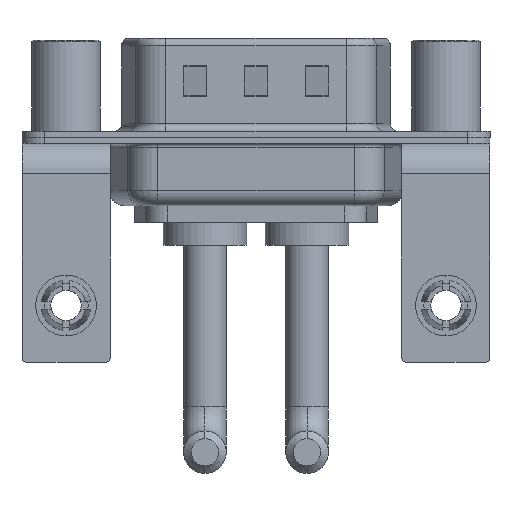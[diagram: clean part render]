
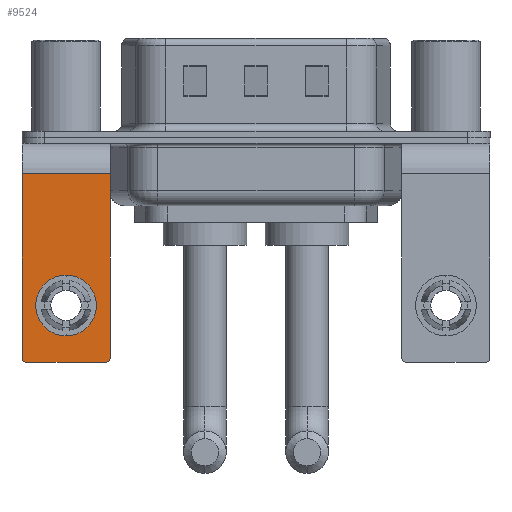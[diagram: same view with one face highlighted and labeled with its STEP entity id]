
A CAD part, front view. The second image highlights one B-rep face of the part: STEP entity #9524.
In plain terms, the highlighted planar face has unit normal (0, -1, 0).
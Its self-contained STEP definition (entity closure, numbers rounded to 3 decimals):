
#386 = DIRECTION ( 'NONE',  ( 0., 0., 1. ) ) ;
#469 = VERTEX_POINT ( 'NONE', #3462 ) ;
#633 = DIRECTION ( 'NONE',  ( -1., 0., 0. ) ) ;
#672 = CARTESIAN_POINT ( 'NONE',  ( 0., -6.25, -13.07 ) ) ;
#917 = AXIS2_PLACEMENT_3D ( 'NONE', #5430, #8339, #12838 ) ;
#1137 = CARTESIAN_POINT ( 'NONE',  ( -2.9, -6.25, -2.4 ) ) ;
#1250 = DIRECTION ( 'NONE',  ( 0., -1., 0. ) ) ;
#1639 = VECTOR ( 'NONE', #633, 1000. ) ;
#1798 = DIRECTION ( 'NONE',  ( 0., 1., 0. ) ) ;
#1852 = LINE ( 'NONE', #17400, #1639 ) ;
#2236 = DIRECTION ( 'NONE',  ( 0., 0., 1. ) ) ;
#2328 = AXIS2_PLACEMENT_3D ( 'NONE', #9857, #1250, #18204 ) ;
#2686 = DIRECTION ( 'NONE',  ( 0., 0., 1. ) ) ;
#3195 = FACE_OUTER_BOUND ( 'NONE', #8102, .T. ) ;
#3323 = DIRECTION ( 'NONE',  ( 0., 0., -1. ) ) ;
#3462 = CARTESIAN_POINT ( 'NONE',  ( -2.9, -6.25, -14.55 ) ) ;
#3502 = VECTOR ( 'NONE', #8519, 1000. ) ;
#3679 = EDGE_CURVE ( 'NONE', #469, #14624, #15259, .T. ) ;
#3863 = ORIENTED_EDGE ( 'NONE', *, *, #17428, .T. ) ;
#3937 = CARTESIAN_POINT ( 'NONE',  ( 2.9, -6.25, -2.4 ) ) ;
#5285 = AXIS2_PLACEMENT_3D ( 'NONE', #15924, #1798, #386 ) ;
#5332 = DIRECTION ( 'NONE',  ( 0., 1., 0. ) ) ;
#5341 = EDGE_CURVE ( 'NONE', #8760, #17216, #17265, .T. ) ;
#5430 = CARTESIAN_POINT ( 'NONE',  ( -2.65, -6.25, -14.55 ) ) ;
#5720 = CARTESIAN_POINT ( 'NONE',  ( -2.9, -6.25, -2.4 ) ) ;
#5729 = AXIS2_PLACEMENT_3D ( 'NONE', #12806, #11202, #2686 ) ;
#5867 = CARTESIAN_POINT ( 'NONE',  ( 0., -6.25, -9.07 ) ) ;
#6025 = VERTEX_POINT ( 'NONE', #3937 ) ;
#6944 = EDGE_CURVE ( 'NONE', #11081, #8406, #16072, .T. ) ;
#7235 = VECTOR ( 'NONE', #3323, 1000. ) ;
#7583 = PLANE ( 'NONE',  #5285 ) ;
#7689 = AXIS2_PLACEMENT_3D ( 'NONE', #18163, #5332, #2236 ) ;
#7928 = ORIENTED_EDGE ( 'NONE', *, *, #11245, .T. ) ;
#8102 = EDGE_LOOP ( 'NONE', ( #7928, #17980, #15222, #12667, #12757, #3863 ) ) ;
#8339 = DIRECTION ( 'NONE',  ( 0., -1., 0. ) ) ;
#8406 = VERTEX_POINT ( 'NONE', #11095 ) ;
#8519 = DIRECTION ( 'NONE',  ( 0., 0., -1. ) ) ;
#8760 = VERTEX_POINT ( 'NONE', #672 ) ;
#9524 = ADVANCED_FACE ( 'NONE', ( #10216, #3195 ), #7583, .F. ) ;
#9753 = CARTESIAN_POINT ( 'NONE',  ( -2.65, -6.25, -14.8 ) ) ;
#9857 = CARTESIAN_POINT ( 'NONE',  ( 2.65, -6.25, -14.55 ) ) ;
#10150 = ORIENTED_EDGE ( 'NONE', *, *, #12179, .T. ) ;
#10216 = FACE_BOUND ( 'NONE', #15599, .T. ) ;
#10690 = VECTOR ( 'NONE', #11944, 1000. ) ;
#11081 = VERTEX_POINT ( 'NONE', #15179 ) ;
#11095 = CARTESIAN_POINT ( 'NONE',  ( 2.9, -6.25, -14.55 ) ) ;
#11202 = DIRECTION ( 'NONE',  ( 0., 1., 0. ) ) ;
#11245 = EDGE_CURVE ( 'NONE', #15941, #469, #15361, .T. ) ;
#11749 = CARTESIAN_POINT ( 'NONE',  ( 2.9, -6.25, -2.4 ) ) ;
#11835 = EDGE_CURVE ( 'NONE', #11081, #14624, #13358, .T. ) ;
#11944 = DIRECTION ( 'NONE',  ( -1., 0., 0. ) ) ;
#12179 = EDGE_CURVE ( 'NONE', #17216, #8760, #16509, .T. ) ;
#12402 = EDGE_CURVE ( 'NONE', #6025, #8406, #13169, .T. ) ;
#12667 = ORIENTED_EDGE ( 'NONE', *, *, #6944, .T. ) ;
#12757 = ORIENTED_EDGE ( 'NONE', *, *, #12402, .F. ) ;
#12806 = CARTESIAN_POINT ( 'NONE',  ( 0., -6.25, -11.07 ) ) ;
#12838 = DIRECTION ( 'NONE',  ( 0., 0., 1. ) ) ;
#13169 = LINE ( 'NONE', #11749, #7235 ) ;
#13267 = CARTESIAN_POINT ( 'NONE',  ( 2.9, -6.25, -14.8 ) ) ;
#13358 = LINE ( 'NONE', #13267, #10690 ) ;
#14624 = VERTEX_POINT ( 'NONE', #9753 ) ;
#15179 = CARTESIAN_POINT ( 'NONE',  ( 2.65, -6.25, -14.8 ) ) ;
#15222 = ORIENTED_EDGE ( 'NONE', *, *, #11835, .F. ) ;
#15259 = CIRCLE ( 'NONE', #917, 0.25 ) ;
#15361 = LINE ( 'NONE', #1137, #3502 ) ;
#15599 = EDGE_LOOP ( 'NONE', ( #17459, #10150 ) ) ;
#15924 = CARTESIAN_POINT ( 'NONE',  ( 2.9, -6.25, -2.4 ) ) ;
#15941 = VERTEX_POINT ( 'NONE', #5720 ) ;
#16072 = CIRCLE ( 'NONE', #2328, 0.25 ) ;
#16509 = CIRCLE ( 'NONE', #5729, 2. ) ;
#17216 = VERTEX_POINT ( 'NONE', #5867 ) ;
#17265 = CIRCLE ( 'NONE', #7689, 2. ) ;
#17400 = CARTESIAN_POINT ( 'NONE',  ( 2.9, -6.25, -2.4 ) ) ;
#17428 = EDGE_CURVE ( 'NONE', #6025, #15941, #1852, .T. ) ;
#17459 = ORIENTED_EDGE ( 'NONE', *, *, #5341, .T. ) ;
#17980 = ORIENTED_EDGE ( 'NONE', *, *, #3679, .T. ) ;
#18163 = CARTESIAN_POINT ( 'NONE',  ( 0., -6.25, -11.07 ) ) ;
#18204 = DIRECTION ( 'NONE',  ( 0., 0., 1. ) ) ;
